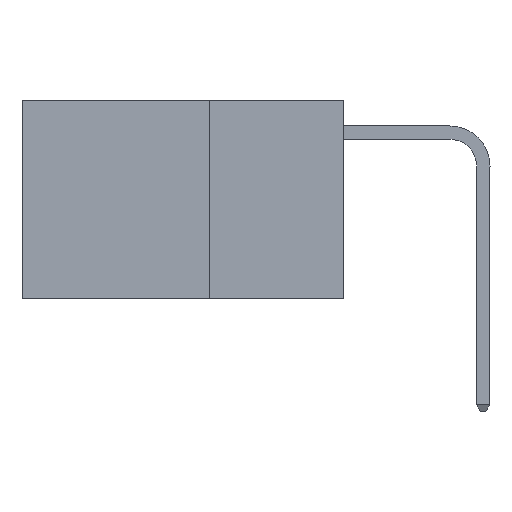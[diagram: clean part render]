
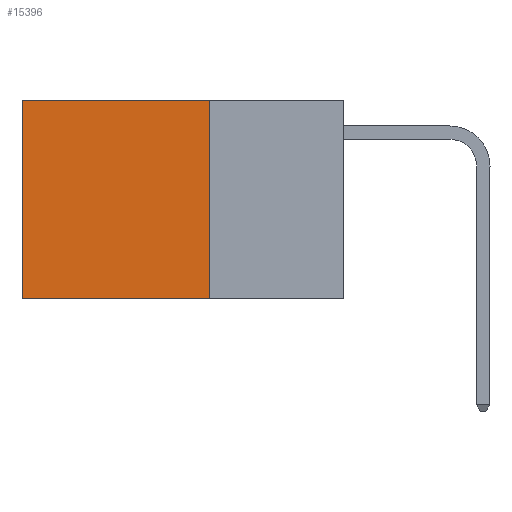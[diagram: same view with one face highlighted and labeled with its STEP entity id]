
A CAD part, left-side view. The second image highlights one B-rep face of the part: STEP entity #15396.
In plain terms, the highlighted planar face has unit normal (-1, 0, 0).
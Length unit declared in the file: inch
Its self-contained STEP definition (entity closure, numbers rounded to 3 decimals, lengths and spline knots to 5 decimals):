
#427 = LINE ( 'NONE', #14145, #10213 ) ;
#1013 = CARTESIAN_POINT ( 'NONE',  ( 0.2625, 0.6, -0.37 ) ) ;
#1425 = EDGE_LOOP ( 'NONE', ( #6218, #6011, #1652, #5649 ) ) ;
#1652 = ORIENTED_EDGE ( 'NONE', *, *, #7647, .F. ) ;
#2796 = DIRECTION ( 'NONE',  ( 0., 0., -1. ) ) ;
#3979 = VERTEX_POINT ( 'NONE', #1013 ) ;
#4023 = CARTESIAN_POINT ( 'NONE',  ( 0.2625, 0.6, 0. ) ) ;
#5407 = CARTESIAN_POINT ( 'NONE',  ( 0.2625, 0.25, -0.37 ) ) ;
#5457 = VERTEX_POINT ( 'NONE', #5407 ) ;
#5649 = ORIENTED_EDGE ( 'NONE', *, *, #14456, .T. ) ;
#5817 = DIRECTION ( 'NONE',  ( 0., 0., -1. ) ) ;
#6011 = ORIENTED_EDGE ( 'NONE', *, *, #7435, .F. ) ;
#6214 = CARTESIAN_POINT ( 'NONE',  ( 0.2625, 0.25, 0. ) ) ;
#6218 = ORIENTED_EDGE ( 'NONE', *, *, #13228, .T. ) ;
#7128 = CARTESIAN_POINT ( 'NONE',  ( 0.2625, 0.25, -0.37 ) ) ;
#7227 = CARTESIAN_POINT ( 'NONE',  ( 0.2625, 0.6, 0. ) ) ;
#7435 = EDGE_CURVE ( 'NONE', #5457, #3979, #13757, .T. ) ;
#7647 = EDGE_CURVE ( 'NONE', #8746, #5457, #13949, .T. ) ;
#7762 = LINE ( 'NONE', #7227, #10853 ) ;
#8057 = CARTESIAN_POINT ( 'NONE',  ( 0.2625, 0.25, 0. ) ) ;
#8315 = FACE_OUTER_BOUND ( 'NONE', #1425, .T. ) ;
#8462 = DIRECTION ( 'NONE',  ( 0., 1., 0. ) ) ;
#8746 = VERTEX_POINT ( 'NONE', #9296 ) ;
#8996 = DIRECTION ( 'NONE',  ( 0., 1., 0. ) ) ;
#9296 = CARTESIAN_POINT ( 'NONE',  ( 0.2625, 0.25, 0. ) ) ;
#10213 = VECTOR ( 'NONE', #8996, 39.37008 ) ;
#10312 = VECTOR ( 'NONE', #8462, 39.37008 ) ;
#10697 = DIRECTION ( 'NONE',  ( 1., 0., 0. ) ) ;
#10853 = VECTOR ( 'NONE', #5817, 39.37008 ) ;
#11774 = VERTEX_POINT ( 'NONE', #4023 ) ;
#11968 = PLANE ( 'NONE',  #14694 ) ;
#13228 = EDGE_CURVE ( 'NONE', #11774, #3979, #7762, .T. ) ;
#13757 = LINE ( 'NONE', #7128, #10312 ) ;
#13949 = LINE ( 'NONE', #6214, #16863 ) ;
#14145 = CARTESIAN_POINT ( 'NONE',  ( 0.2625, 0.25, 0. ) ) ;
#14456 = EDGE_CURVE ( 'NONE', #8746, #11774, #427, .T. ) ;
#14694 = AXIS2_PLACEMENT_3D ( 'NONE', #8057, #10697, #2796 ) ;
#15396 = ADVANCED_FACE ( 'NONE', ( #8315 ), #11968, .F. ) ;
#16524 = DIRECTION ( 'NONE',  ( 0., 0., -1. ) ) ;
#16863 = VECTOR ( 'NONE', #16524, 39.37008 ) ;
